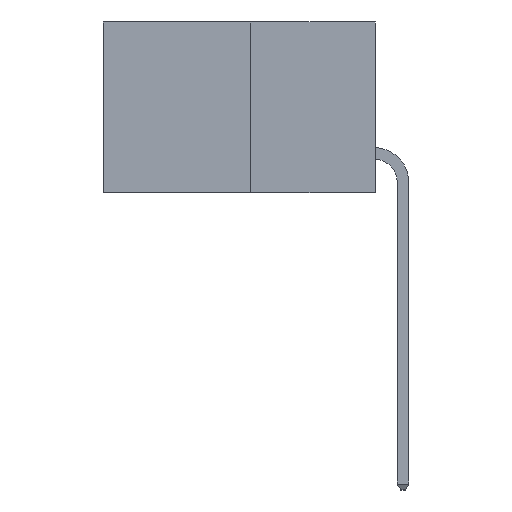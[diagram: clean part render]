
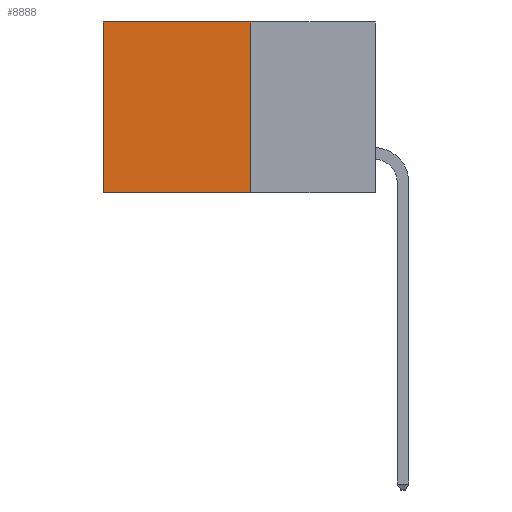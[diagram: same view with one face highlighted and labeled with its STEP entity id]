
A CAD part, left-side view. The second image highlights one B-rep face of the part: STEP entity #8888.
In plain terms, the highlighted planar face has unit normal (-1, 0, 0).
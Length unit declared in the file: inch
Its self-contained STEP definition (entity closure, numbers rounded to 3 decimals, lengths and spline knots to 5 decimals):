
#40 = CARTESIAN_POINT ( 'NONE',  ( 0.277, 0.27, 0. ) ) ;
#1189 = VECTOR ( 'NONE', #4477, 39.37008 ) ;
#2523 = DIRECTION ( 'NONE',  ( 0., 1., 0. ) ) ;
#3290 = VECTOR ( 'NONE', #8158, 39.37008 ) ;
#3489 = CARTESIAN_POINT ( 'NONE',  ( 0.277, 0.27, -0.37 ) ) ;
#3860 = VERTEX_POINT ( 'NONE', #12058 ) ;
#3910 = LINE ( 'NONE', #8419, #6621 ) ;
#4105 = CARTESIAN_POINT ( 'NONE',  ( 0.277, 0.27, 0. ) ) ;
#4216 = FACE_OUTER_BOUND ( 'NONE', #8657, .T. ) ;
#4477 = DIRECTION ( 'NONE',  ( 0., 0., -1. ) ) ;
#4636 = DIRECTION ( 'NONE',  ( 1., 0., 0. ) ) ;
#5250 = VERTEX_POINT ( 'NONE', #11579 ) ;
#6234 = VECTOR ( 'NONE', #2523, 39.37008 ) ;
#6466 = EDGE_CURVE ( 'NONE', #3860, #5250, #3910, .T. ) ;
#6621 = VECTOR ( 'NONE', #9628, 39.37008 ) ;
#6673 = VERTEX_POINT ( 'NONE', #4105 ) ;
#6749 = AXIS2_PLACEMENT_3D ( 'NONE', #10417, #4636, #12744 ) ;
#7499 = LINE ( 'NONE', #9077, #1189 ) ;
#8125 = PLANE ( 'NONE',  #6749 ) ;
#8158 = DIRECTION ( 'NONE',  ( 0., 1., 0. ) ) ;
#8238 = CARTESIAN_POINT ( 'NONE',  ( 0.277, 0.27, -0.37 ) ) ;
#8419 = CARTESIAN_POINT ( 'NONE',  ( 0.277, 0.59, -0.37 ) ) ;
#8657 = EDGE_LOOP ( 'NONE', ( #12168, #10541, #11344, #11471 ) ) ;
#8888 = ADVANCED_FACE ( 'NONE', ( #4216 ), #8125, .F. ) ;
#9077 = CARTESIAN_POINT ( 'NONE',  ( 0.277, 0.27, -0.37 ) ) ;
#9381 = LINE ( 'NONE', #40, #6234 ) ;
#9530 = LINE ( 'NONE', #3489, #3290 ) ;
#9628 = DIRECTION ( 'NONE',  ( 0., 0., -1. ) ) ;
#10155 = VERTEX_POINT ( 'NONE', #8238 ) ;
#10226 = EDGE_CURVE ( 'NONE', #6673, #3860, #9381, .T. ) ;
#10417 = CARTESIAN_POINT ( 'NONE',  ( 0.277, 0.27, -0.37 ) ) ;
#10541 = ORIENTED_EDGE ( 'NONE', *, *, #11298, .F. ) ;
#11298 = EDGE_CURVE ( 'NONE', #10155, #5250, #9530, .T. ) ;
#11344 = ORIENTED_EDGE ( 'NONE', *, *, #11686, .F. ) ;
#11471 = ORIENTED_EDGE ( 'NONE', *, *, #10226, .T. ) ;
#11579 = CARTESIAN_POINT ( 'NONE',  ( 0.277, 0.59, -0.37 ) ) ;
#11686 = EDGE_CURVE ( 'NONE', #6673, #10155, #7499, .T. ) ;
#12058 = CARTESIAN_POINT ( 'NONE',  ( 0.277, 0.59, 0. ) ) ;
#12168 = ORIENTED_EDGE ( 'NONE', *, *, #6466, .T. ) ;
#12744 = DIRECTION ( 'NONE',  ( 0., 0., -1. ) ) ;
